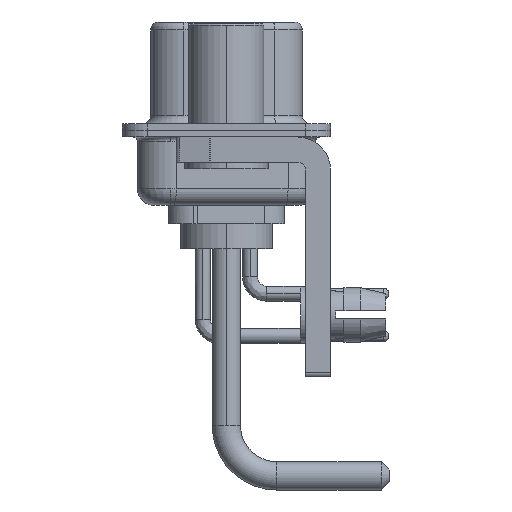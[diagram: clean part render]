
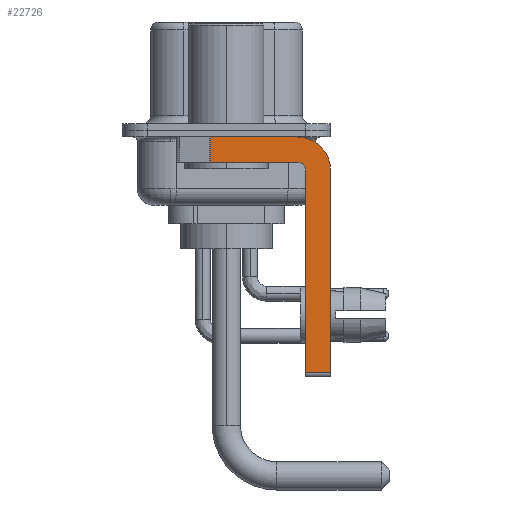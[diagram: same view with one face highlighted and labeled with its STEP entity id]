
A CAD part, left-side view. The second image highlights one B-rep face of the part: STEP entity #22726.
In plain terms, the highlighted planar face has unit normal (-1, 0, 0).
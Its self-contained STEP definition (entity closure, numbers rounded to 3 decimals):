
#638 = VECTOR ( 'NONE', #27164, 1000. ) ;
#664 = DIRECTION ( 'NONE',  ( 0., 0., 1. ) ) ;
#1061 = FACE_OUTER_BOUND ( 'NONE', #1098, .T. ) ;
#1098 = EDGE_LOOP ( 'NONE', ( #21132, #16355, #24987, #22808, #10664, #8583, #24012, #18296 ) ) ;
#1192 = EDGE_CURVE ( 'NONE', #22411, #24203, #4329, .T. ) ;
#1784 = EDGE_CURVE ( 'NONE', #22685, #10564, #7176, .T. ) ;
#2066 = VECTOR ( 'NONE', #5285, 1000. ) ;
#2832 = CARTESIAN_POINT ( 'NONE',  ( -2.9, -4.75, -14.8 ) ) ;
#3133 = EDGE_CURVE ( 'NONE', #22742, #8066, #24875, .T. ) ;
#3243 = AXIS2_PLACEMENT_3D ( 'NONE', #18719, #3934, #14933 ) ;
#3934 = DIRECTION ( 'NONE',  ( 1., 0., 0. ) ) ;
#4085 = VERTEX_POINT ( 'NONE', #21107 ) ;
#4329 = CIRCLE ( 'NONE', #14863, 2. ) ;
#4428 = EDGE_CURVE ( 'NONE', #22685, #4085, #18746, .T. ) ;
#5285 = DIRECTION ( 'NONE',  ( 0., -1., 0. ) ) ;
#5601 = CARTESIAN_POINT ( 'NONE',  ( -2.9, -4.25, -2.4 ) ) ;
#5702 = CARTESIAN_POINT ( 'NONE',  ( -2.9, -4.25, -14.55 ) ) ;
#6712 = CARTESIAN_POINT ( 'NONE',  ( -2.9, -4.25, -0.4 ) ) ;
#7176 = LINE ( 'NONE', #2832, #22851 ) ;
#7862 = DIRECTION ( 'NONE',  ( -1., 0., 0. ) ) ;
#8066 = VERTEX_POINT ( 'NONE', #14735 ) ;
#8583 = ORIENTED_EDGE ( 'NONE', *, *, #4428, .T. ) ;
#8909 = CARTESIAN_POINT ( 'NONE',  ( -2.9, -4.25, -1.9 ) ) ;
#9104 = VECTOR ( 'NONE', #10128, 1000. ) ;
#9583 = CIRCLE ( 'NONE', #10482, 0.5 ) ;
#9891 = PLANE ( 'NONE',  #3243 ) ;
#10128 = DIRECTION ( 'NONE',  ( 0., 0., -1. ) ) ;
#10172 = CARTESIAN_POINT ( 'NONE',  ( -2.9, -4.75, -14.55 ) ) ;
#10409 = CARTESIAN_POINT ( 'NONE',  ( -2.9, -6.25, -2.4 ) ) ;
#10482 = AXIS2_PLACEMENT_3D ( 'NONE', #14225, #7862, #16687 ) ;
#10564 = VERTEX_POINT ( 'NONE', #16026 ) ;
#10664 = ORIENTED_EDGE ( 'NONE', *, *, #1784, .F. ) ;
#14005 = DIRECTION ( 'NONE',  ( 1., 0., 0. ) ) ;
#14225 = CARTESIAN_POINT ( 'NONE',  ( -2.9, -4.25, -2.4 ) ) ;
#14391 = EDGE_CURVE ( 'NONE', #22620, #8066, #18313, .T. ) ;
#14735 = CARTESIAN_POINT ( 'NONE',  ( -2.9, 0.978, -1.9 ) ) ;
#14863 = AXIS2_PLACEMENT_3D ( 'NONE', #5601, #14005, #25011 ) ;
#14933 = DIRECTION ( 'NONE',  ( 0., 0., -1. ) ) ;
#15030 = VECTOR ( 'NONE', #19174, 1000. ) ;
#15669 = EDGE_CURVE ( 'NONE', #22742, #22411, #15714, .T. ) ;
#15714 = LINE ( 'NONE', #22389, #2066 ) ;
#15748 = CARTESIAN_POINT ( 'NONE',  ( -2.9, 0.978, -1.9 ) ) ;
#16026 = CARTESIAN_POINT ( 'NONE',  ( -2.9, -4.75, -2.4 ) ) ;
#16355 = ORIENTED_EDGE ( 'NONE', *, *, #3133, .T. ) ;
#16687 = DIRECTION ( 'NONE',  ( 0., 0., 1. ) ) ;
#17247 = CARTESIAN_POINT ( 'NONE',  ( -2.9, 0.978, -0.4 ) ) ;
#17716 = EDGE_CURVE ( 'NONE', #10564, #22620, #9583, .T. ) ;
#17975 = EDGE_CURVE ( 'NONE', #24203, #4085, #25765, .T. ) ;
#18296 = ORIENTED_EDGE ( 'NONE', *, *, #1192, .F. ) ;
#18313 = LINE ( 'NONE', #8909, #638 ) ;
#18719 = CARTESIAN_POINT ( 'NONE',  ( -2.9, -4.25, -2.4 ) ) ;
#18746 = LINE ( 'NONE', #5702, #15030 ) ;
#19174 = DIRECTION ( 'NONE',  ( 0., -1., 0. ) ) ;
#20904 = CARTESIAN_POINT ( 'NONE',  ( -2.9, -4.25, -1.9 ) ) ;
#21107 = CARTESIAN_POINT ( 'NONE',  ( -2.9, -6.25, -14.55 ) ) ;
#21132 = ORIENTED_EDGE ( 'NONE', *, *, #15669, .F. ) ;
#22380 = VECTOR ( 'NONE', #25021, 1000. ) ;
#22389 = CARTESIAN_POINT ( 'NONE',  ( -2.9, 3., -0.4 ) ) ;
#22411 = VERTEX_POINT ( 'NONE', #6712 ) ;
#22620 = VERTEX_POINT ( 'NONE', #20904 ) ;
#22685 = VERTEX_POINT ( 'NONE', #10172 ) ;
#22726 = ADVANCED_FACE ( 'NONE', ( #1061 ), #9891, .F. ) ;
#22742 = VERTEX_POINT ( 'NONE', #17247 ) ;
#22808 = ORIENTED_EDGE ( 'NONE', *, *, #17716, .F. ) ;
#22851 = VECTOR ( 'NONE', #664, 1000. ) ;
#24012 = ORIENTED_EDGE ( 'NONE', *, *, #17975, .F. ) ;
#24203 = VERTEX_POINT ( 'NONE', #25560 ) ;
#24875 = LINE ( 'NONE', #15748, #22380 ) ;
#24987 = ORIENTED_EDGE ( 'NONE', *, *, #14391, .F. ) ;
#25011 = DIRECTION ( 'NONE',  ( 0., 0., -1. ) ) ;
#25021 = DIRECTION ( 'NONE',  ( 0., 0., -1. ) ) ;
#25560 = CARTESIAN_POINT ( 'NONE',  ( -2.9, -6.25, -2.4 ) ) ;
#25765 = LINE ( 'NONE', #10409, #9104 ) ;
#27164 = DIRECTION ( 'NONE',  ( 0., 1., 0. ) ) ;
